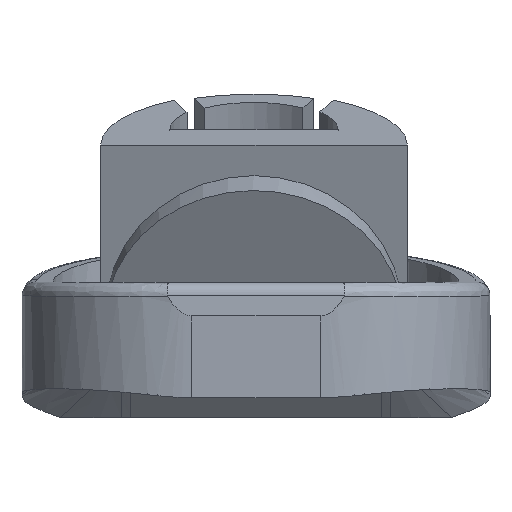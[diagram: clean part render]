
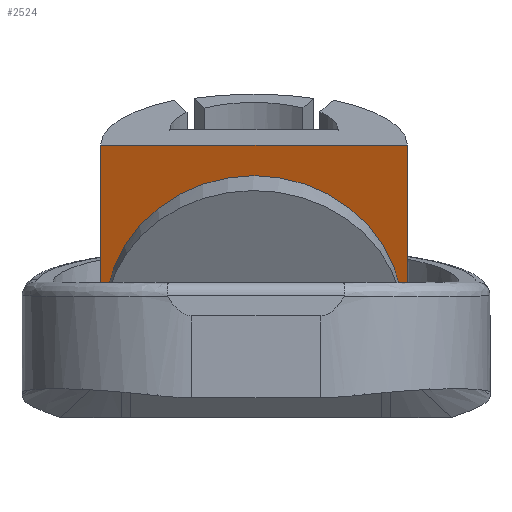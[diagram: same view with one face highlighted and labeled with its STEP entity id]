
A CAD part, left-side view. The second image highlights one B-rep face of the part: STEP entity #2524.
In plain terms, the highlighted planar face has unit normal (-0.94, 0, -0.342).
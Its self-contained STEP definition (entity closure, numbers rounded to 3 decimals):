
#178=CIRCLE('',#2556,11.);
#372=FACE_OUTER_BOUND('',#510,.T.);
#510=EDGE_LOOP('',(#2289,#2290,#2291,#2292,#2293,#2294));
#539=LINE('',#3370,#710);
#544=LINE('',#3389,#715);
#685=LINE('',#6250,#856);
#686=LINE('',#6254,#857);
#687=LINE('',#6255,#858);
#710=VECTOR('',#2801,10.);
#715=VECTOR('',#2816,10.);
#856=VECTOR('',#3269,10.);
#857=VECTOR('',#3274,10.);
#858=VECTOR('',#3275,10.);
#933=VERTEX_POINT('',#3322);
#934=VERTEX_POINT('',#3323);
#955=VERTEX_POINT('',#3369);
#964=VERTEX_POINT('',#3387);
#1173=VERTEX_POINT('',#6249);
#1174=VERTEX_POINT('',#6253);
#1186=EDGE_CURVE('',#933,#934,#178,.T.);
#1209=EDGE_CURVE('',#933,#955,#539,.T.);
#1219=EDGE_CURVE('',#964,#934,#544,.T.);
#1553=EDGE_CURVE('',#964,#1173,#685,.T.);
#1555=EDGE_CURVE('',#1174,#1173,#686,.T.);
#1556=EDGE_CURVE('',#1174,#955,#687,.T.);
#2289=ORIENTED_EDGE('',*,*,#1186,.T.);
#2290=ORIENTED_EDGE('',*,*,#1219,.F.);
#2291=ORIENTED_EDGE('',*,*,#1553,.T.);
#2292=ORIENTED_EDGE('',*,*,#1555,.F.);
#2293=ORIENTED_EDGE('',*,*,#1556,.T.);
#2294=ORIENTED_EDGE('',*,*,#1209,.F.);
#2389=PLANE('',#2729);
#2524=ADVANCED_FACE('',(#372),#2389,.T.);
#2556=AXIS2_PLACEMENT_3D('',#3324,#2765,#2766);
#2729=AXIS2_PLACEMENT_3D('',#6252,#3272,#3273);
#2765=DIRECTION('center_axis',(0.94,0.,0.342));
#2766=DIRECTION('ref_axis',(-0.342,0.,0.94));
#2801=DIRECTION('',(0.,1.,0.));
#2816=DIRECTION('',(0.,1.,0.));
#3269=DIRECTION('',(-0.342,0.,0.94));
#3272=DIRECTION('center_axis',(-0.94,0.,-0.342));
#3273=DIRECTION('ref_axis',(0.,1.,0.));
#3274=DIRECTION('',(0.,-1.,0.));
#3275=DIRECTION('',(0.342,0.,-0.94));
#3322=CARTESIAN_POINT('',(58.454,32.,5.));
#3323=CARTESIAN_POINT('',(58.454,10.,5.));
#3324=CARTESIAN_POINT('Origin',(58.454,21.,5.));
#3369=CARTESIAN_POINT('',(58.454,32.3,5.));
#3370=CARTESIAN_POINT('',(58.454,15.275,5.));
#3387=CARTESIAN_POINT('',(58.454,9.7,5.));
#3389=CARTESIAN_POINT('',(58.454,15.275,5.));
#6249=CARTESIAN_POINT('',(53.87,9.7,17.595));
#6250=CARTESIAN_POINT('',(55.067,9.7,14.306));
#6252=CARTESIAN_POINT('Origin',(55.067,9.7,14.306));
#6253=CARTESIAN_POINT('',(53.87,32.3,17.595));
#6254=CARTESIAN_POINT('',(53.87,32.,17.595));
#6255=CARTESIAN_POINT('',(55.067,32.3,14.306));
